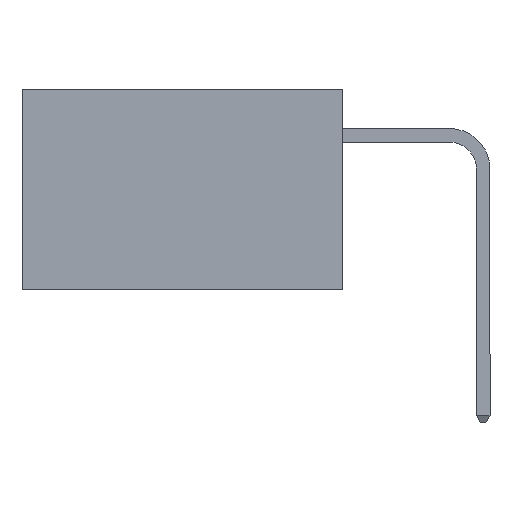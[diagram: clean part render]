
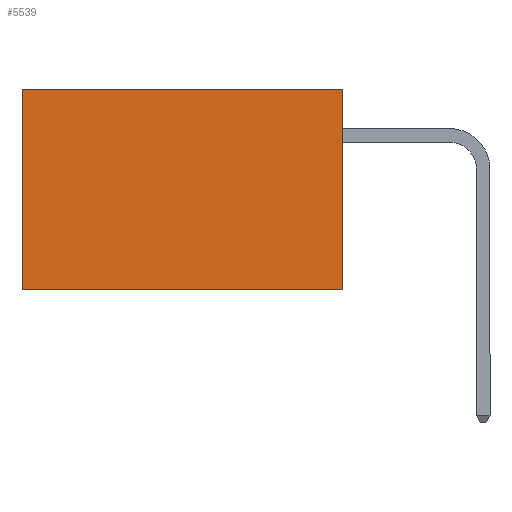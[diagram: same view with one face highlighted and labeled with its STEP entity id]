
A CAD part, left-side view. The second image highlights one B-rep face of the part: STEP entity #5539.
In plain terms, the highlighted planar face has unit normal (-1, 0, 0).
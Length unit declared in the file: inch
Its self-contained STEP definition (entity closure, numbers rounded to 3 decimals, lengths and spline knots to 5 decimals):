
#104 = CARTESIAN_POINT ( 'NONE',  ( 0.277, 0., -0.37 ) ) ;
#106 = PLANE ( 'NONE',  #4526 ) ;
#481 = ORIENTED_EDGE ( 'NONE', *, *, #4255, .F. ) ;
#810 = VECTOR ( 'NONE', #2837, 39.37008 ) ;
#1386 = DIRECTION ( 'NONE',  ( 0., 0., -1. ) ) ;
#1398 = DIRECTION ( 'NONE',  ( 1., 0., 0. ) ) ;
#1534 = LINE ( 'NONE', #4185, #3094 ) ;
#1960 = CARTESIAN_POINT ( 'NONE',  ( 0.277, 0.59, -0.37 ) ) ;
#2072 = VERTEX_POINT ( 'NONE', #2510 ) ;
#2115 = EDGE_CURVE ( 'NONE', #2072, #4014, #3719, .T. ) ;
#2219 = VERTEX_POINT ( 'NONE', #1960 ) ;
#2237 = ORIENTED_EDGE ( 'NONE', *, *, #2115, .T. ) ;
#2510 = CARTESIAN_POINT ( 'NONE',  ( 0.277, 0., 0. ) ) ;
#2837 = DIRECTION ( 'NONE',  ( 0., 0., -1. ) ) ;
#2878 = CARTESIAN_POINT ( 'NONE',  ( 0.277, 0.59, -0.37 ) ) ;
#3094 = VECTOR ( 'NONE', #4484, 39.37008 ) ;
#3719 = LINE ( 'NONE', #6194, #6717 ) ;
#3735 = ORIENTED_EDGE ( 'NONE', *, *, #6506, .T. ) ;
#3808 = CARTESIAN_POINT ( 'NONE',  ( 0.277, 0., -0.37 ) ) ;
#4014 = VERTEX_POINT ( 'NONE', #5899 ) ;
#4185 = CARTESIAN_POINT ( 'NONE',  ( 0.277, 0., -0.37 ) ) ;
#4255 = EDGE_CURVE ( 'NONE', #2072, #4343, #7420, .T. ) ;
#4343 = VERTEX_POINT ( 'NONE', #3808 ) ;
#4379 = EDGE_CURVE ( 'NONE', #4343, #2219, #1534, .T. ) ;
#4484 = DIRECTION ( 'NONE',  ( 0., 1., 0. ) ) ;
#4526 = AXIS2_PLACEMENT_3D ( 'NONE', #104, #1398, #1386 ) ;
#4997 = EDGE_LOOP ( 'NONE', ( #3735, #5369, #481, #2237 ) ) ;
#5369 = ORIENTED_EDGE ( 'NONE', *, *, #4379, .F. ) ;
#5539 = ADVANCED_FACE ( 'NONE', ( #6491 ), #106, .F. ) ;
#5888 = VECTOR ( 'NONE', #7273, 39.37008 ) ;
#5899 = CARTESIAN_POINT ( 'NONE',  ( 0.277, 0.59, 0. ) ) ;
#6143 = DIRECTION ( 'NONE',  ( 0., 1., 0. ) ) ;
#6194 = CARTESIAN_POINT ( 'NONE',  ( 0.277, 0., 0. ) ) ;
#6491 = FACE_OUTER_BOUND ( 'NONE', #4997, .T. ) ;
#6506 = EDGE_CURVE ( 'NONE', #4014, #2219, #7392, .T. ) ;
#6717 = VECTOR ( 'NONE', #6143, 39.37008 ) ;
#7273 = DIRECTION ( 'NONE',  ( 0., 0., -1. ) ) ;
#7392 = LINE ( 'NONE', #2878, #810 ) ;
#7420 = LINE ( 'NONE', #7749, #5888 ) ;
#7749 = CARTESIAN_POINT ( 'NONE',  ( 0.277, 0., -0.37 ) ) ;
